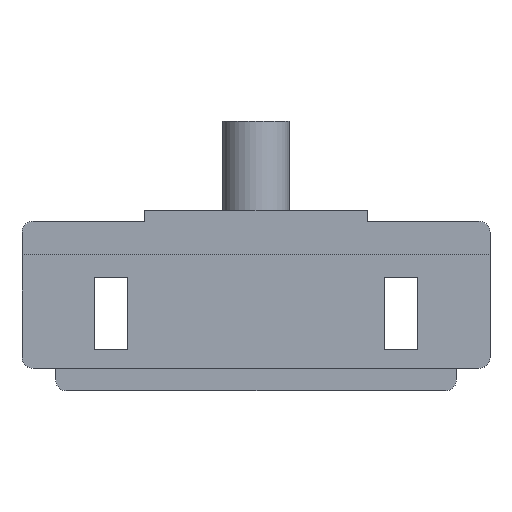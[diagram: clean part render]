
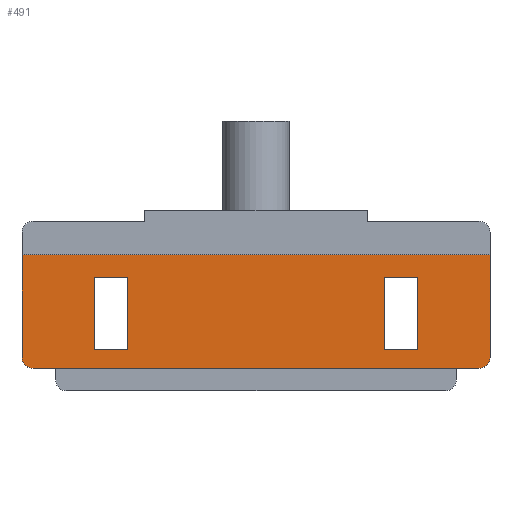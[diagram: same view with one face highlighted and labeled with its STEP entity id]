
A CAD part, top view. The second image highlights one B-rep face of the part: STEP entity #491.
In plain terms, the highlighted planar face has unit normal (0, 0, 1).
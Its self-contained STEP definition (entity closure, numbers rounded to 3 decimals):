
#19 = ORIENTED_EDGE ( 'NONE', *, *, #423, .F. ) ;
#54 = VECTOR ( 'NONE', #69, 1000. ) ;
#66 = EDGE_CURVE ( 'NONE', #271, #888, #501, .T. ) ;
#67 = DIRECTION ( 'NONE',  ( -1., 0., 0. ) ) ;
#69 = DIRECTION ( 'NONE',  ( 0., 1., 0. ) ) ;
#71 = CARTESIAN_POINT ( 'NONE',  ( -106.3, 8.693, -25.1 ) ) ;
#77 = ORIENTED_EDGE ( 'NONE', *, *, #546, .F. ) ;
#85 = AXIS2_PLACEMENT_3D ( 'NONE', #317, #1178, #320 ) ;
#95 = EDGE_CURVE ( 'NONE', #1191, #1200, #440, .T. ) ;
#101 = CARTESIAN_POINT ( 'NONE',  ( -80.3, 6.293, -25.1 ) ) ;
#107 = VECTOR ( 'NONE', #330, 1000. ) ;
#130 = DIRECTION ( 'NONE',  ( 0., 0., -1. ) ) ;
#156 = CARTESIAN_POINT ( 'NONE',  ( -109.8, 4.593, -25.1 ) ) ;
#159 = LINE ( 'NONE', #1324, #1280 ) ;
#162 = CARTESIAN_POINT ( 'NONE',  ( -112.8, 14.793, -25.1 ) ) ;
#183 = CARTESIAN_POINT ( 'NONE',  ( -111.8, 5.593, -25.1 ) ) ;
#195 = LINE ( 'NONE', #595, #54 ) ;
#200 = CARTESIAN_POINT ( 'NONE',  ( -70.8, 5.593, -25.1 ) ) ;
#205 = ORIENTED_EDGE ( 'NONE', *, *, #1022, .F. ) ;
#210 = VECTOR ( 'NONE', #918, 1000. ) ;
#212 = VECTOR ( 'NONE', #675, 1000. ) ;
#246 = CARTESIAN_POINT ( 'NONE',  ( -77.3, 6.293, -25.1 ) ) ;
#255 = VERTEX_POINT ( 'NONE', #1102 ) ;
#257 = VECTOR ( 'NONE', #676, 1000. ) ;
#267 = EDGE_LOOP ( 'NONE', ( #304, #958, #526, #19 ) ) ;
#271 = VERTEX_POINT ( 'NONE', #200 ) ;
#273 = DIRECTION ( 'NONE',  ( 1., 0., 0. ) ) ;
#282 = DIRECTION ( 'NONE',  ( 0., -1., 0. ) ) ;
#304 = ORIENTED_EDGE ( 'NONE', *, *, #413, .F. ) ;
#314 = LINE ( 'NONE', #71, #982 ) ;
#317 = CARTESIAN_POINT ( 'NONE',  ( -70.8, 4.593, -25.1 ) ) ;
#320 = DIRECTION ( 'NONE',  ( 1., 0., 0. ) ) ;
#323 = VECTOR ( 'NONE', #1069, 1000. ) ;
#330 = DIRECTION ( 'NONE',  ( -1., 0., 0. ) ) ;
#346 = EDGE_CURVE ( 'NONE', #671, #408, #1053, .T. ) ;
#378 = LINE ( 'NONE', #390, #1202 ) ;
#380 = DIRECTION ( 'NONE',  ( 1., 0., 0. ) ) ;
#390 = CARTESIAN_POINT ( 'NONE',  ( -112.8, 4.593, -25.1 ) ) ;
#391 = ORIENTED_EDGE ( 'NONE', *, *, #640, .T. ) ;
#392 = DIRECTION ( 'NONE',  ( 1., 0., 0. ) ) ;
#405 = LINE ( 'NONE', #1171, #323 ) ;
#407 = LINE ( 'NONE', #932, #769 ) ;
#408 = VERTEX_POINT ( 'NONE', #1268 ) ;
#412 = ORIENTED_EDGE ( 'NONE', *, *, #346, .T. ) ;
#413 = EDGE_CURVE ( 'NONE', #951, #556, #1168, .T. ) ;
#423 = EDGE_CURVE ( 'NONE', #556, #1191, #314, .T. ) ;
#426 = CARTESIAN_POINT ( 'NONE',  ( -112.8, 4.593, -25.1 ) ) ;
#434 = AXIS2_PLACEMENT_3D ( 'NONE', #183, #713, #67 ) ;
#440 = LINE ( 'NONE', #553, #212 ) ;
#455 = LINE ( 'NONE', #608, #1198 ) ;
#473 = ORIENTED_EDGE ( 'NONE', *, *, #1086, .T. ) ;
#481 = EDGE_CURVE ( 'NONE', #1130, #1062, #941, .T. ) ;
#491 = ADVANCED_FACE ( 'NONE', ( #880, #560, #1181 ), #1393, .F. ) ;
#496 = LINE ( 'NONE', #1343, #210 ) ;
#501 = CIRCLE ( 'NONE', #899, 1. ) ;
#510 = CARTESIAN_POINT ( 'NONE',  ( -87.05, 12.793, -25.1 ) ) ;
#525 = VERTEX_POINT ( 'NONE', #101 ) ;
#526 = ORIENTED_EDGE ( 'NONE', *, *, #95, .F. ) ;
#536 = ORIENTED_EDGE ( 'NONE', *, *, #1275, .T. ) ;
#546 = EDGE_CURVE ( 'NONE', #986, #525, #405, .T. ) ;
#553 = CARTESIAN_POINT ( 'NONE',  ( -88.55, 6.293, -25.1 ) ) ;
#556 = VERTEX_POINT ( 'NONE', #942 ) ;
#560 = FACE_BOUND ( 'NONE', #980, .T. ) ;
#562 = CARTESIAN_POINT ( 'NONE',  ( -74.05, 12.793, -25.1 ) ) ;
#591 = VERTEX_POINT ( 'NONE', #162 ) ;
#592 = EDGE_CURVE ( 'NONE', #408, #1130, #455, .T. ) ;
#595 = CARTESIAN_POINT ( 'NONE',  ( -77.3, 5.443, -25.1 ) ) ;
#608 = CARTESIAN_POINT ( 'NONE',  ( -112.8, 4.593, -25.1 ) ) ;
#624 = EDGE_CURVE ( 'NONE', #1200, #951, #496, .T. ) ;
#633 = EDGE_CURVE ( 'NONE', #710, #255, #195, .T. ) ;
#640 = EDGE_CURVE ( 'NONE', #591, #671, #407, .T. ) ;
#642 = ORIENTED_EDGE ( 'NONE', *, *, #66, .F. ) ;
#646 = VECTOR ( 'NONE', #965, 1000. ) ;
#652 = CARTESIAN_POINT ( 'NONE',  ( -103.3, 12.793, -25.1 ) ) ;
#656 = ORIENTED_EDGE ( 'NONE', *, *, #1162, .F. ) ;
#671 = VERTEX_POINT ( 'NONE', #1313 ) ;
#675 = DIRECTION ( 'NONE',  ( 1., 0., 0. ) ) ;
#676 = DIRECTION ( 'NONE',  ( -1., 0., 0. ) ) ;
#710 = VERTEX_POINT ( 'NONE', #246 ) ;
#713 = DIRECTION ( 'NONE',  ( 0., 0., 1. ) ) ;
#727 = DIRECTION ( 'NONE',  ( -1., 0., 0. ) ) ;
#756 = VERTEX_POINT ( 'NONE', #1320 ) ;
#769 = VECTOR ( 'NONE', #282, 1000. ) ;
#802 = EDGE_LOOP ( 'NONE', ( #997, #1044, #473, #642, #536, #1346, #391, #412 ) ) ;
#880 = FACE_OUTER_BOUND ( 'NONE', #802, .T. ) ;
#881 = DIRECTION ( 'NONE',  ( -1., 0., 0. ) ) ;
#888 = VERTEX_POINT ( 'NONE', #1299 ) ;
#899 = AXIS2_PLACEMENT_3D ( 'NONE', #1205, #130, #881 ) ;
#918 = DIRECTION ( 'NONE',  ( 0., 1., 0. ) ) ;
#919 = VECTOR ( 'NONE', #273, 1000. ) ;
#932 = CARTESIAN_POINT ( 'NONE',  ( -112.8, 14.793, -25.1 ) ) ;
#940 = CARTESIAN_POINT ( 'NONE',  ( -73.8, 4.593, -25.1 ) ) ;
#941 = LINE ( 'NONE', #426, #646 ) ;
#942 = CARTESIAN_POINT ( 'NONE',  ( -106.3, 12.793, -25.1 ) ) ;
#946 = DIRECTION ( 'NONE',  ( 0., -1., 0. ) ) ;
#948 = CARTESIAN_POINT ( 'NONE',  ( -106.3, 6.293, -25.1 ) ) ;
#951 = VERTEX_POINT ( 'NONE', #652 ) ;
#958 = ORIENTED_EDGE ( 'NONE', *, *, #624, .F. ) ;
#959 = EDGE_CURVE ( 'NONE', #756, #591, #1258, .T. ) ;
#965 = DIRECTION ( 'NONE',  ( 1., 0., 0. ) ) ;
#980 = EDGE_LOOP ( 'NONE', ( #205, #1377, #656, #77 ) ) ;
#982 = VECTOR ( 'NONE', #946, 1000. ) ;
#986 = VERTEX_POINT ( 'NONE', #1396 ) ;
#987 = LINE ( 'NONE', #562, #257 ) ;
#997 = ORIENTED_EDGE ( 'NONE', *, *, #592, .T. ) ;
#1022 = EDGE_CURVE ( 'NONE', #255, #986, #987, .T. ) ;
#1044 = ORIENTED_EDGE ( 'NONE', *, *, #481, .T. ) ;
#1052 = CARTESIAN_POINT ( 'NONE',  ( -103.3, 6.293, -25.1 ) ) ;
#1053 = CIRCLE ( 'NONE', #434, 1. ) ;
#1062 = VERTEX_POINT ( 'NONE', #940 ) ;
#1069 = DIRECTION ( 'NONE',  ( 0., -1., 0. ) ) ;
#1080 = CARTESIAN_POINT ( 'NONE',  ( -70.8, 14.793, -25.1 ) ) ;
#1086 = EDGE_CURVE ( 'NONE', #1062, #888, #378, .T. ) ;
#1098 = VECTOR ( 'NONE', #727, 1000. ) ;
#1102 = CARTESIAN_POINT ( 'NONE',  ( -77.3, 12.793, -25.1 ) ) ;
#1130 = VERTEX_POINT ( 'NONE', #156 ) ;
#1162 = EDGE_CURVE ( 'NONE', #525, #710, #1238, .T. ) ;
#1168 = LINE ( 'NONE', #510, #1098 ) ;
#1171 = CARTESIAN_POINT ( 'NONE',  ( -80.3, 8.693, -25.1 ) ) ;
#1178 = DIRECTION ( 'NONE',  ( 0., 0., -1. ) ) ;
#1181 = FACE_BOUND ( 'NONE', #267, .T. ) ;
#1191 = VERTEX_POINT ( 'NONE', #948 ) ;
#1198 = VECTOR ( 'NONE', #392, 1000. ) ;
#1200 = VERTEX_POINT ( 'NONE', #1052 ) ;
#1202 = VECTOR ( 'NONE', #380, 1000. ) ;
#1205 = CARTESIAN_POINT ( 'NONE',  ( -71.8, 5.593, -25.1 ) ) ;
#1238 = LINE ( 'NONE', #1368, #919 ) ;
#1258 = LINE ( 'NONE', #1080, #107 ) ;
#1268 = CARTESIAN_POINT ( 'NONE',  ( -111.8, 4.593, -25.1 ) ) ;
#1275 = EDGE_CURVE ( 'NONE', #271, #756, #159, .T. ) ;
#1280 = VECTOR ( 'NONE', #1332, 1000. ) ;
#1299 = CARTESIAN_POINT ( 'NONE',  ( -71.8, 4.593, -25.1 ) ) ;
#1313 = CARTESIAN_POINT ( 'NONE',  ( -112.8, 5.593, -25.1 ) ) ;
#1320 = CARTESIAN_POINT ( 'NONE',  ( -70.8, 14.793, -25.1 ) ) ;
#1324 = CARTESIAN_POINT ( 'NONE',  ( -70.8, 4.593, -25.1 ) ) ;
#1332 = DIRECTION ( 'NONE',  ( 0., 1., 0. ) ) ;
#1343 = CARTESIAN_POINT ( 'NONE',  ( -103.3, 5.443, -25.1 ) ) ;
#1346 = ORIENTED_EDGE ( 'NONE', *, *, #959, .T. ) ;
#1368 = CARTESIAN_POINT ( 'NONE',  ( -75.55, 6.293, -25.1 ) ) ;
#1377 = ORIENTED_EDGE ( 'NONE', *, *, #633, .F. ) ;
#1393 = PLANE ( 'NONE',  #85 ) ;
#1396 = CARTESIAN_POINT ( 'NONE',  ( -80.3, 12.793, -25.1 ) ) ;
